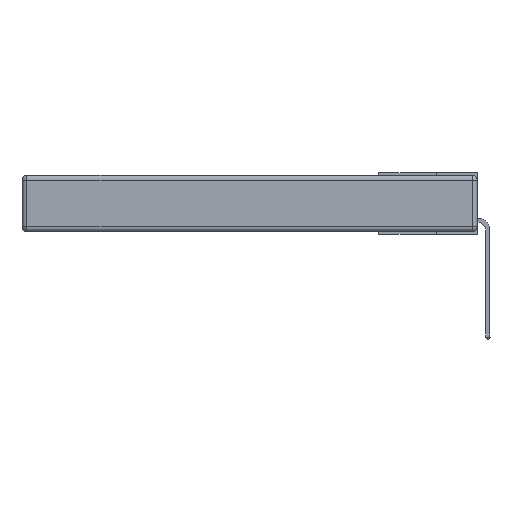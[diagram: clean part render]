
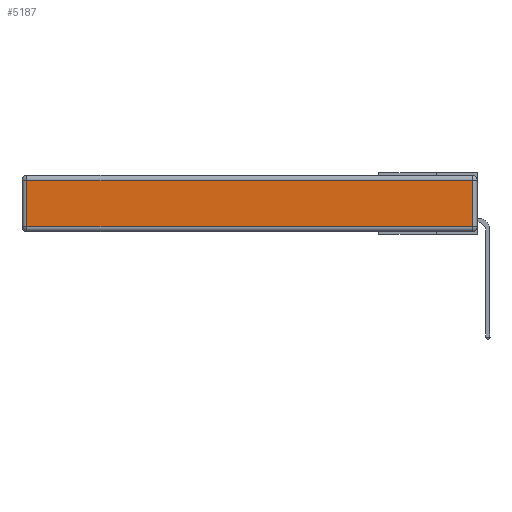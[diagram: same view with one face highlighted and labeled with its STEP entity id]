
A CAD part, left-side view. The second image highlights one B-rep face of the part: STEP entity #5187.
In plain terms, the highlighted planar face has unit normal (-1, 0, 0).
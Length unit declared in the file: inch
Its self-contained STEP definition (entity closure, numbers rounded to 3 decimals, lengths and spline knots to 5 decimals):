
#1439 = VERTEX_POINT ( 'NONE', #9235 ) ;
#1700 = CARTESIAN_POINT ( 'NONE',  ( 0., 2.72, -0.343 ) ) ;
#2351 = LINE ( 'NONE', #4276, #12562 ) ;
#2377 = VECTOR ( 'NONE', #10506, 39.37008 ) ;
#2477 = VECTOR ( 'NONE', #5024, 39.37008 ) ;
#2592 = CARTESIAN_POINT ( 'NONE',  ( 0., 0.03, -0.313 ) ) ;
#2717 = FACE_OUTER_BOUND ( 'NONE', #9770, .T. ) ;
#2996 = VERTEX_POINT ( 'NONE', #2592 ) ;
#4276 = CARTESIAN_POINT ( 'NONE',  ( 0., 0.03, -0.343 ) ) ;
#4780 = EDGE_CURVE ( 'NONE', #2996, #9947, #2351, .T. ) ;
#5024 = DIRECTION ( 'NONE',  ( 0., 1., 0. ) ) ;
#5176 = EDGE_CURVE ( 'NONE', #1439, #2996, #14934, .T. ) ;
#5187 = ADVANCED_FACE ( 'NONE', ( #2717 ), #5412, .T. ) ;
#5412 = PLANE ( 'NONE',  #15261 ) ;
#5507 = VERTEX_POINT ( 'NONE', #12146 ) ;
#5809 = ORIENTED_EDGE ( 'NONE', *, *, #6990, .T. ) ;
#6387 = CARTESIAN_POINT ( 'NONE',  ( 0., 0., -0.313 ) ) ;
#6721 = ORIENTED_EDGE ( 'NONE', *, *, #16248, .T. ) ;
#6990 = EDGE_CURVE ( 'NONE', #9947, #5507, #10924, .T. ) ;
#7364 = CARTESIAN_POINT ( 'NONE',  ( 0., 2.75, -0.03 ) ) ;
#8076 = LINE ( 'NONE', #1700, #2377 ) ;
#8613 = VECTOR ( 'NONE', #11438, 39.37008 ) ;
#8962 = ORIENTED_EDGE ( 'NONE', *, *, #4780, .T. ) ;
#9110 = CARTESIAN_POINT ( 'NONE',  ( 0., 0., -0.343 ) ) ;
#9235 = CARTESIAN_POINT ( 'NONE',  ( 0., 2.72, -0.313 ) ) ;
#9770 = EDGE_LOOP ( 'NONE', ( #10286, #8962, #5809, #6721 ) ) ;
#9947 = VERTEX_POINT ( 'NONE', #11572 ) ;
#10286 = ORIENTED_EDGE ( 'NONE', *, *, #5176, .T. ) ;
#10327 = DIRECTION ( 'NONE',  ( -1., 0., 0. ) ) ;
#10506 = DIRECTION ( 'NONE',  ( 0., 0., -1. ) ) ;
#10924 = LINE ( 'NONE', #7364, #2477 ) ;
#11438 = DIRECTION ( 'NONE',  ( 0., -1., 0. ) ) ;
#11572 = CARTESIAN_POINT ( 'NONE',  ( 0., 0.03, -0.03 ) ) ;
#11784 = DIRECTION ( 'NONE',  ( 0., 0., 1. ) ) ;
#12146 = CARTESIAN_POINT ( 'NONE',  ( 0., 2.72, -0.03 ) ) ;
#12562 = VECTOR ( 'NONE', #11784, 39.37008 ) ;
#12806 = DIRECTION ( 'NONE',  ( 0., 0., 1. ) ) ;
#14934 = LINE ( 'NONE', #6387, #8613 ) ;
#15261 = AXIS2_PLACEMENT_3D ( 'NONE', #9110, #10327, #12806 ) ;
#16248 = EDGE_CURVE ( 'NONE', #5507, #1439, #8076, .T. ) ;
